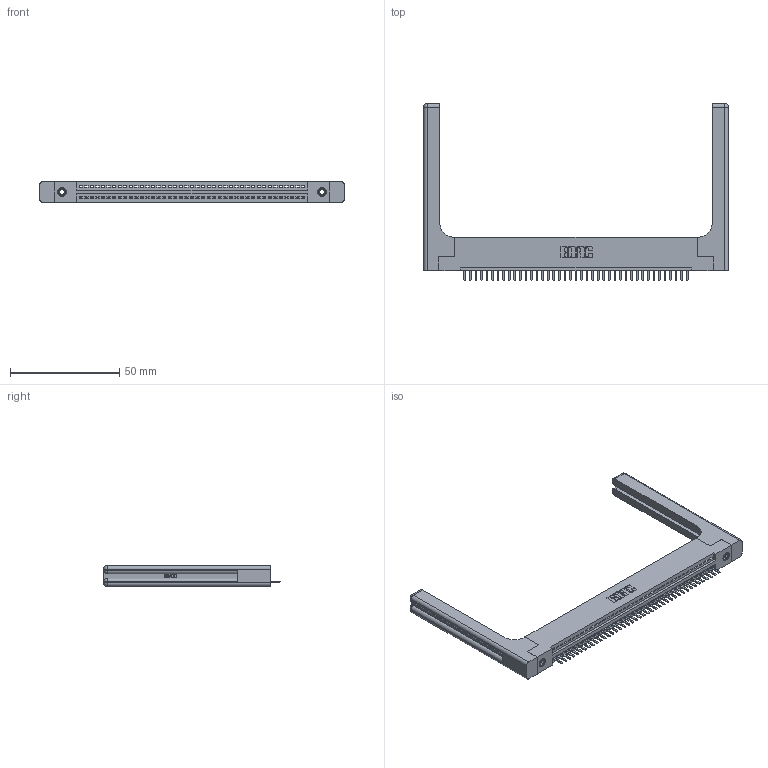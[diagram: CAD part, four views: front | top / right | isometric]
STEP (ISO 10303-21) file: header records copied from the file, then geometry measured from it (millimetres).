
FILE_DESCRIPTION (( 'STEP AP203' ), '1' );
FILE_NAME ('395-041-520-158.STEP', '2019-10-22T06:23:03', ( '' ), ( '' ), 'SwSTEP 2.0', 'SolidWorks 2016', '' );
FILE_SCHEMA (( 'CONFIG_CONTROL_DESIGN' ));
Length unit declared in the file: inch
Products named in the file (5): 345 Part_Flush Mounting Lugs - 0.156 Dia-TH; 395-041-520-158; 345-220-058_345-220-058; 345-292-001_345-293-120; 345-250-001_345-250-001-102
Assembly tree (46 placements, depth 2):
  395-041-520-158
    345 Part_Flush Mounting Lugs - 0.156 Dia-TH
    345-292-001_345-293-120  x41
    345-250-001_345-250-001-102  x2
    345-220-058_345-220-058  x2
Bounding box: 139.17 x 80.64 x 9.4 mm (x, y, z)
Volume: 21597 mm3; surface area: 22304.3 mm2
Topology: 46 solids, 46 shells, 2924 faces, 8551 edges, 5570 vertices
Faces by surface type: plane 1950, cylinder 914, bspline 36, cone 12, sphere 8, torus 4
Entity records: 36288 total; most frequent: CARTESIAN_POINT 7268, ORIENTED_EDGE 6028, DIRECTION 5284, EDGE_CURVE 3014, LINE 2622, VECTOR 2622, VERTEX_POINT 1998, AXIS2_PLACEMENT_3D 1331
